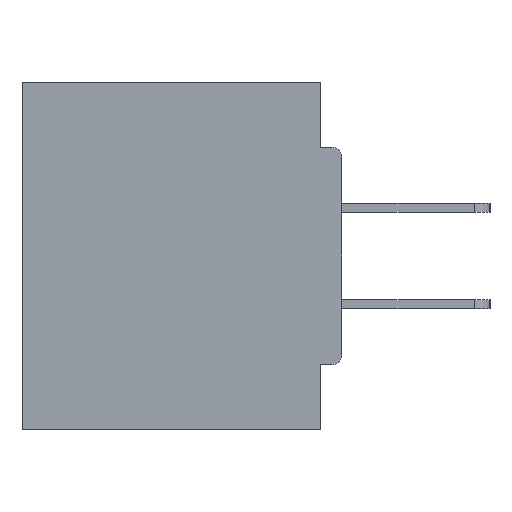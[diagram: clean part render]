
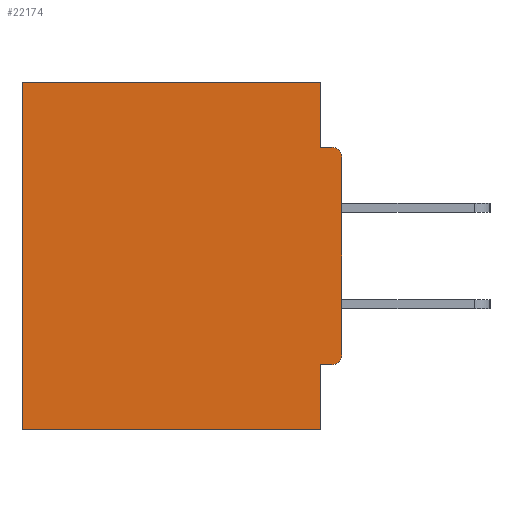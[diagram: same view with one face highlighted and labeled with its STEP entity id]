
A CAD part, left-side view. The second image highlights one B-rep face of the part: STEP entity #22174.
In plain terms, the highlighted planar face has unit normal (-1, 0, 0).
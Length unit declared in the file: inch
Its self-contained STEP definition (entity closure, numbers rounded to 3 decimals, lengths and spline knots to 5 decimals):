
#1039 = VERTEX_POINT ( 'NONE', #30287 ) ;
#1238 = CARTESIAN_POINT ( 'NONE',  ( 0.298, 0., -0.4065 ) ) ;
#1542 = ORIENTED_EDGE ( 'NONE', *, *, #11926, .T. ) ;
#2207 = CARTESIAN_POINT ( 'NONE',  ( 0.298, 0.46, 0. ) ) ;
#2444 = VECTOR ( 'NONE', #31591, 39.37008 ) ;
#2859 = AXIS2_PLACEMENT_3D ( 'NONE', #14910, #29513, #3559 ) ;
#3559 = DIRECTION ( 'NONE',  ( 0., 0., -1. ) ) ;
#4255 = CIRCLE ( 'NONE', #25741, 0.015 ) ;
#4498 = DIRECTION ( 'NONE',  ( 0., 1., 0. ) ) ;
#4503 = EDGE_LOOP ( 'NONE', ( #32944, #27346, #5761, #15934, #1542, #21053, #35588, #32058, #6077, #20887 ) ) ;
#4863 = DIRECTION ( 'NONE',  ( 0., 0., -1. ) ) ;
#5224 = EDGE_CURVE ( 'NONE', #14143, #1039, #4255, .T. ) ;
#5447 = CARTESIAN_POINT ( 'NONE',  ( 0.298, 0.031, -0.5 ) ) ;
#5515 = VECTOR ( 'NONE', #16418, 39.37008 ) ;
#5761 = ORIENTED_EDGE ( 'NONE', *, *, #31012, .F. ) ;
#6077 = ORIENTED_EDGE ( 'NONE', *, *, #6287, .T. ) ;
#6287 = EDGE_CURVE ( 'NONE', #10733, #16925, #16644, .T. ) ;
#8040 = DIRECTION ( 'NONE',  ( -1., 0., 0. ) ) ;
#9150 = VECTOR ( 'NONE', #4863, 39.37008 ) ;
#9308 = VECTOR ( 'NONE', #4498, 39.37008 ) ;
#9404 = CARTESIAN_POINT ( 'NONE',  ( 0.298, 0.46, -0.5 ) ) ;
#9948 = PLANE ( 'NONE',  #10337 ) ;
#10316 = CARTESIAN_POINT ( 'NONE',  ( 0.298, 0., 0. ) ) ;
#10337 = AXIS2_PLACEMENT_3D ( 'NONE', #10316, #27331, #33037 ) ;
#10733 = VERTEX_POINT ( 'NONE', #35867 ) ;
#11599 = CARTESIAN_POINT ( 'NONE',  ( 0.298, 0.46, 0. ) ) ;
#11926 = EDGE_CURVE ( 'NONE', #12163, #19213, #30846, .T. ) ;
#12163 = VERTEX_POINT ( 'NONE', #11599 ) ;
#13190 = VECTOR ( 'NONE', #14324, 39.37008 ) ;
#14143 = VERTEX_POINT ( 'NONE', #22303 ) ;
#14324 = DIRECTION ( 'NONE',  ( 0., 0., -1. ) ) ;
#14499 = EDGE_CURVE ( 'NONE', #22221, #19213, #28128, .T. ) ;
#14910 = CARTESIAN_POINT ( 'NONE',  ( 0.298, 0.015, -0.3915 ) ) ;
#15317 = FACE_OUTER_BOUND ( 'NONE', #4503, .T. ) ;
#15321 = CARTESIAN_POINT ( 'NONE',  ( 0.298, 0.031, -0.0935 ) ) ;
#15567 = EDGE_CURVE ( 'NONE', #14143, #16925, #28492, .T. ) ;
#15934 = ORIENTED_EDGE ( 'NONE', *, *, #22417, .T. ) ;
#16418 = DIRECTION ( 'NONE',  ( 0., -1., 0. ) ) ;
#16644 = CIRCLE ( 'NONE', #2859, 0.015 ) ;
#16925 = VERTEX_POINT ( 'NONE', #33083 ) ;
#17764 = CARTESIAN_POINT ( 'NONE',  ( 0.298, 0., 0. ) ) ;
#17859 = CARTESIAN_POINT ( 'NONE',  ( 0.298, 0., -0.5 ) ) ;
#19213 = VERTEX_POINT ( 'NONE', #9404 ) ;
#19439 = CARTESIAN_POINT ( 'NONE',  ( 0.298, 0.031, 0. ) ) ;
#20266 = DIRECTION ( 'NONE',  ( 0., 0., -1. ) ) ;
#20887 = ORIENTED_EDGE ( 'NONE', *, *, #15567, .F. ) ;
#20896 = EDGE_CURVE ( 'NONE', #25216, #1039, #34374, .T. ) ;
#21053 = ORIENTED_EDGE ( 'NONE', *, *, #14499, .F. ) ;
#21102 = LINE ( 'NONE', #17764, #31526 ) ;
#21539 = VERTEX_POINT ( 'NONE', #30301 ) ;
#22145 = CARTESIAN_POINT ( 'NONE',  ( 0.298, 0., -0.0935 ) ) ;
#22174 = ADVANCED_FACE ( 'NONE', ( #15317 ), #9948, .F. ) ;
#22221 = VERTEX_POINT ( 'NONE', #24426 ) ;
#22303 = CARTESIAN_POINT ( 'NONE',  ( 0.298, 0., -0.1085 ) ) ;
#22417 = EDGE_CURVE ( 'NONE', #34147, #12163, #21102, .T. ) ;
#22683 = VECTOR ( 'NONE', #26770, 39.37008 ) ;
#22980 = CARTESIAN_POINT ( 'NONE',  ( 0.298, 0.031, -0.5 ) ) ;
#23865 = EDGE_CURVE ( 'NONE', #10733, #21539, #32341, .T. ) ;
#24426 = CARTESIAN_POINT ( 'NONE',  ( 0.298, 0.031, -0.5 ) ) ;
#25216 = VERTEX_POINT ( 'NONE', #15321 ) ;
#25741 = AXIS2_PLACEMENT_3D ( 'NONE', #26936, #8040, #20266 ) ;
#26770 = DIRECTION ( 'NONE',  ( 0., 1., 0. ) ) ;
#26936 = CARTESIAN_POINT ( 'NONE',  ( 0.298, 0.015, -0.1085 ) ) ;
#27331 = DIRECTION ( 'NONE',  ( 1., 0., 0. ) ) ;
#27346 = ORIENTED_EDGE ( 'NONE', *, *, #20896, .F. ) ;
#28128 = LINE ( 'NONE', #17859, #22683 ) ;
#28492 = LINE ( 'NONE', #32008, #13190 ) ;
#28731 = DIRECTION ( 'NONE',  ( 0., 0., -1. ) ) ;
#29503 = LINE ( 'NONE', #22980, #2444 ) ;
#29513 = DIRECTION ( 'NONE',  ( -1., 0., 0. ) ) ;
#30287 = CARTESIAN_POINT ( 'NONE',  ( 0.298, 0.015, -0.0935 ) ) ;
#30301 = CARTESIAN_POINT ( 'NONE',  ( 0.298, 0.031, -0.4065 ) ) ;
#30584 = LINE ( 'NONE', #5447, #32850 ) ;
#30846 = LINE ( 'NONE', #2207, #9150 ) ;
#31012 = EDGE_CURVE ( 'NONE', #34147, #25216, #30584, .T. ) ;
#31526 = VECTOR ( 'NONE', #34900, 39.37008 ) ;
#31591 = DIRECTION ( 'NONE',  ( 0., 0., -1. ) ) ;
#32008 = CARTESIAN_POINT ( 'NONE',  ( 0.298, 0., 0. ) ) ;
#32058 = ORIENTED_EDGE ( 'NONE', *, *, #23865, .F. ) ;
#32341 = LINE ( 'NONE', #1238, #9308 ) ;
#32537 = EDGE_CURVE ( 'NONE', #21539, #22221, #29503, .T. ) ;
#32850 = VECTOR ( 'NONE', #28731, 39.37008 ) ;
#32944 = ORIENTED_EDGE ( 'NONE', *, *, #5224, .T. ) ;
#33037 = DIRECTION ( 'NONE',  ( 0., 0., -1. ) ) ;
#33083 = CARTESIAN_POINT ( 'NONE',  ( 0.298, 0., -0.3915 ) ) ;
#34147 = VERTEX_POINT ( 'NONE', #19439 ) ;
#34374 = LINE ( 'NONE', #22145, #5515 ) ;
#34900 = DIRECTION ( 'NONE',  ( 0., 1., 0. ) ) ;
#35588 = ORIENTED_EDGE ( 'NONE', *, *, #32537, .F. ) ;
#35867 = CARTESIAN_POINT ( 'NONE',  ( 0.298, 0.015, -0.4065 ) ) ;
